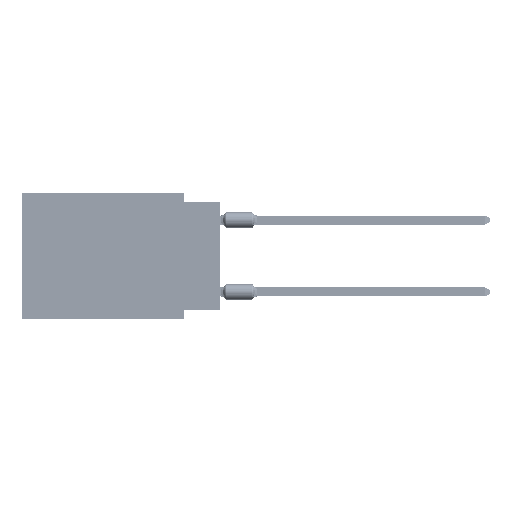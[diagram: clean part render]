
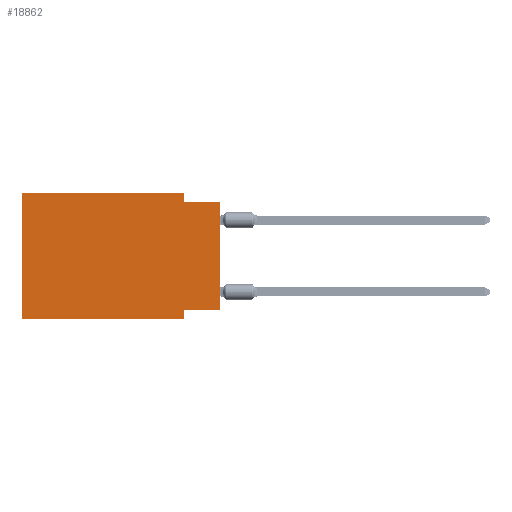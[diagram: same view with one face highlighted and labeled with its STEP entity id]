
A CAD part, left-side view. The second image highlights one B-rep face of the part: STEP entity #18862.
In plain terms, the highlighted planar face has unit normal (-1, 0, 0).
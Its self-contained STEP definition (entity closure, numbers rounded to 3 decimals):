
#2742 = LINE ( 'NONE', #37676, #55035 ) ;
#5182 = EDGE_CURVE ( 'NONE', #48065, #11787, #18594, .T. ) ;
#5941 = EDGE_CURVE ( 'NONE', #33321, #76206, #50589, .T. ) ;
#6402 = EDGE_CURVE ( 'NONE', #51967, #46163, #29612, .T. ) ;
#7313 = VECTOR ( 'NONE', #11727, 1000. ) ;
#8611 = DIRECTION ( 'NONE',  ( 0., -1., 0. ) ) ;
#8862 = DIRECTION ( 'NONE',  ( 0., 0., 1. ) ) ;
#9192 = EDGE_CURVE ( 'NONE', #51967, #32970, #24443, .T. ) ;
#11727 = DIRECTION ( 'NONE',  ( 0., 0., -1. ) ) ;
#11787 = VERTEX_POINT ( 'NONE', #46638 ) ;
#14846 = AXIS2_PLACEMENT_3D ( 'NONE', #81996, #19104, #55389 ) ;
#15353 = ORIENTED_EDGE ( 'NONE', *, *, #80377, .F. ) ;
#15688 = VECTOR ( 'NONE', #8611, 1000. ) ;
#15917 = CARTESIAN_POINT ( 'NONE',  ( 0., 2.54, -8.255 ) ) ;
#17075 = CARTESIAN_POINT ( 'NONE',  ( 0., 2.54, 0. ) ) ;
#17140 = VERTEX_POINT ( 'NONE', #88115 ) ;
#17166 = ORIENTED_EDGE ( 'NONE', *, *, #29543, .F. ) ;
#18594 = LINE ( 'NONE', #73699, #27789 ) ;
#18862 = ADVANCED_FACE ( 'NONE', ( #63187 ), #27361, .F. ) ;
#19104 = DIRECTION ( 'NONE',  ( 1., 0., 0. ) ) ;
#19147 = ORIENTED_EDGE ( 'NONE', *, *, #5182, .T. ) ;
#19536 = CARTESIAN_POINT ( 'NONE',  ( 0., 2.54, -0.635 ) ) ;
#23176 = DIRECTION ( 'NONE',  ( 0., 1., 0. ) ) ;
#23853 = VECTOR ( 'NONE', #8862, 1000. ) ;
#24072 = CARTESIAN_POINT ( 'NONE',  ( 0., 0., -8.255 ) ) ;
#24443 = LINE ( 'NONE', #64904, #23853 ) ;
#27361 = PLANE ( 'NONE',  #14846 ) ;
#27789 = VECTOR ( 'NONE', #31465, 1000. ) ;
#28078 = DIRECTION ( 'NONE',  ( 0., 0., -1. ) ) ;
#28700 = ORIENTED_EDGE ( 'NONE', *, *, #34993, .F. ) ;
#29241 = VECTOR ( 'NONE', #23176, 1000. ) ;
#29296 = ORIENTED_EDGE ( 'NONE', *, *, #6402, .F. ) ;
#29543 = EDGE_CURVE ( 'NONE', #48065, #17140, #2742, .T. ) ;
#29612 = LINE ( 'NONE', #24072, #29241 ) ;
#31465 = DIRECTION ( 'NONE',  ( 0., -1., 0. ) ) ;
#32970 = VERTEX_POINT ( 'NONE', #89687 ) ;
#33321 = VERTEX_POINT ( 'NONE', #17075 ) ;
#34993 = EDGE_CURVE ( 'NONE', #46163, #11787, #87525, .T. ) ;
#36019 = EDGE_CURVE ( 'NONE', #76206, #32970, #46892, .T. ) ;
#37676 = CARTESIAN_POINT ( 'NONE',  ( 0., 13.97, 0. ) ) ;
#38028 = VECTOR ( 'NONE', #28078, 1000. ) ;
#39771 = ORIENTED_EDGE ( 'NONE', *, *, #9192, .T. ) ;
#43711 = CARTESIAN_POINT ( 'NONE',  ( 0., 2.54, 0. ) ) ;
#46163 = VERTEX_POINT ( 'NONE', #15917 ) ;
#46638 = CARTESIAN_POINT ( 'NONE',  ( 0., 2.54, -8.89 ) ) ;
#46892 = LINE ( 'NONE', #90008, #79290 ) ;
#48065 = VERTEX_POINT ( 'NONE', #76529 ) ;
#50589 = LINE ( 'NONE', #43711, #38028 ) ;
#51967 = VERTEX_POINT ( 'NONE', #81158 ) ;
#55035 = VECTOR ( 'NONE', #73007, 1000. ) ;
#55131 = DIRECTION ( 'NONE',  ( 0., -1., 0. ) ) ;
#55389 = DIRECTION ( 'NONE',  ( 0., 0., -1. ) ) ;
#56864 = CARTESIAN_POINT ( 'NONE',  ( 0., 13.97, 0. ) ) ;
#63187 = FACE_OUTER_BOUND ( 'NONE', #89331, .T. ) ;
#64904 = CARTESIAN_POINT ( 'NONE',  ( 0., 0., 0. ) ) ;
#67891 = LINE ( 'NONE', #56864, #15688 ) ;
#73007 = DIRECTION ( 'NONE',  ( 0., 0., 1. ) ) ;
#73699 = CARTESIAN_POINT ( 'NONE',  ( 0., 13.97, -8.89 ) ) ;
#76206 = VERTEX_POINT ( 'NONE', #19536 ) ;
#76529 = CARTESIAN_POINT ( 'NONE',  ( 0., 13.97, -8.89 ) ) ;
#79290 = VECTOR ( 'NONE', #55131, 1000. ) ;
#79359 = ORIENTED_EDGE ( 'NONE', *, *, #36019, .F. ) ;
#79569 = ORIENTED_EDGE ( 'NONE', *, *, #5941, .F. ) ;
#80377 = EDGE_CURVE ( 'NONE', #17140, #33321, #67891, .T. ) ;
#81158 = CARTESIAN_POINT ( 'NONE',  ( 0., 0., -8.255 ) ) ;
#81996 = CARTESIAN_POINT ( 'NONE',  ( 0., 13.97, 0. ) ) ;
#87065 = CARTESIAN_POINT ( 'NONE',  ( 0., 2.54, -8.89 ) ) ;
#87525 = LINE ( 'NONE', #87065, #7313 ) ;
#88115 = CARTESIAN_POINT ( 'NONE',  ( 0., 13.97, 0. ) ) ;
#89331 = EDGE_LOOP ( 'NONE', ( #39771, #79359, #79569, #15353, #17166, #19147, #28700, #29296 ) ) ;
#89687 = CARTESIAN_POINT ( 'NONE',  ( 0., 0., -0.635 ) ) ;
#90008 = CARTESIAN_POINT ( 'NONE',  ( 0., 0., -0.635 ) ) ;
